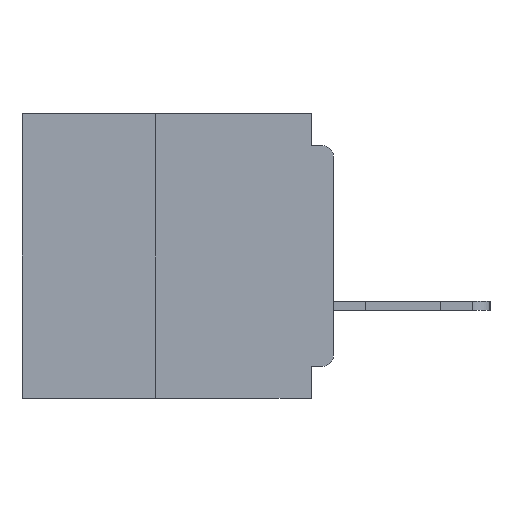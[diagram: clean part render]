
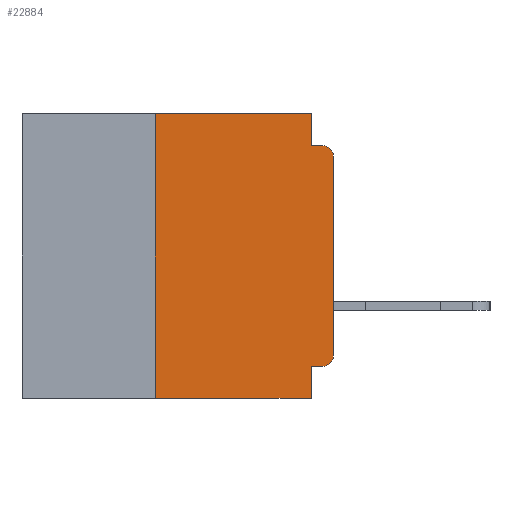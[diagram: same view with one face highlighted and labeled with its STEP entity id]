
A CAD part, left-side view. The second image highlights one B-rep face of the part: STEP entity #22884.
In plain terms, the highlighted planar face has unit normal (-1, 0, 0).
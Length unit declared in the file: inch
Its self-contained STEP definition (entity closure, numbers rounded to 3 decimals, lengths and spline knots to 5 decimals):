
#156 = VECTOR ( 'NONE', #20571, 39.37008 ) ;
#613 = CARTESIAN_POINT ( 'NONE',  ( 0., 0.031, 0. ) ) ;
#863 = ORIENTED_EDGE ( 'NONE', *, *, #7558, .F. ) ;
#2432 = DIRECTION ( 'NONE',  ( 0., -1., 0. ) ) ;
#2804 = LINE ( 'NONE', #26421, #23518 ) ;
#2999 = AXIS2_PLACEMENT_3D ( 'NONE', #21089, #50036, #25255 ) ;
#4055 = CARTESIAN_POINT ( 'NONE',  ( 0., 0., -0.045 ) ) ;
#5027 = PLANE ( 'NONE',  #18846 ) ;
#5218 = DIRECTION ( 'NONE',  ( 1., 0., 0. ) ) ;
#6605 = DIRECTION ( 'NONE',  ( 0., 0., -1. ) ) ;
#7536 = LINE ( 'NONE', #10752, #28291 ) ;
#7558 = EDGE_CURVE ( 'NONE', #16709, #9457, #7536, .T. ) ;
#7922 = VECTOR ( 'NONE', #2432, 39.37008 ) ;
#8011 = DIRECTION ( 'NONE',  ( 0., -1., 0. ) ) ;
#8352 = LINE ( 'NONE', #15480, #40159 ) ;
#8773 = VERTEX_POINT ( 'NONE', #31298 ) ;
#9457 = VERTEX_POINT ( 'NONE', #48027 ) ;
#10752 = CARTESIAN_POINT ( 'NONE',  ( 0., 0.031, 0. ) ) ;
#10824 = VECTOR ( 'NONE', #41363, 39.37008 ) ;
#13518 = EDGE_CURVE ( 'NONE', #9457, #46432, #51888, .T. ) ;
#14701 = VERTEX_POINT ( 'NONE', #28368 ) ;
#15480 = CARTESIAN_POINT ( 'NONE',  ( 0., 0.25, -0.4 ) ) ;
#16709 = VERTEX_POINT ( 'NONE', #613 ) ;
#17668 = LINE ( 'NONE', #27251, #7922 ) ;
#18846 = AXIS2_PLACEMENT_3D ( 'NONE', #30014, #5218, #34219 ) ;
#18885 = VECTOR ( 'NONE', #8011, 39.37008 ) ;
#19050 = CIRCLE ( 'NONE', #39985, 0.015 ) ;
#20107 = VERTEX_POINT ( 'NONE', #28566 ) ;
#20383 = DIRECTION ( 'NONE',  ( 0., 1., 0. ) ) ;
#20571 = DIRECTION ( 'NONE',  ( 0., 0., 1. ) ) ;
#20787 = DIRECTION ( 'NONE',  ( -1., 0., 0. ) ) ;
#21089 = CARTESIAN_POINT ( 'NONE',  ( 0., 0.015, -0.34 ) ) ;
#21862 = LINE ( 'NONE', #53591, #10824 ) ;
#22233 = CARTESIAN_POINT ( 'NONE',  ( 0., 0.031, -0.355 ) ) ;
#22884 = ADVANCED_FACE ( 'NONE', ( #32968 ), #5027, .F. ) ;
#23518 = VECTOR ( 'NONE', #30559, 39.37008 ) ;
#24378 = ORIENTED_EDGE ( 'NONE', *, *, #25657, .T. ) ;
#24441 = ORIENTED_EDGE ( 'NONE', *, *, #44058, .T. ) ;
#25255 = DIRECTION ( 'NONE',  ( 0., 0., -1. ) ) ;
#25657 = EDGE_CURVE ( 'NONE', #14701, #8773, #30044, .T. ) ;
#26421 = CARTESIAN_POINT ( 'NONE',  ( 0., 0.437, -0.4 ) ) ;
#27190 = CARTESIAN_POINT ( 'NONE',  ( 0., 0.031, -0.4 ) ) ;
#27251 = CARTESIAN_POINT ( 'NONE',  ( 0., 0.437, 0. ) ) ;
#28291 = VECTOR ( 'NONE', #6605, 39.37008 ) ;
#28368 = CARTESIAN_POINT ( 'NONE',  ( 0., 0.015, -0.355 ) ) ;
#28566 = CARTESIAN_POINT ( 'NONE',  ( 0., 0.25, -0.4 ) ) ;
#30014 = CARTESIAN_POINT ( 'NONE',  ( 0., 0.437, 0. ) ) ;
#30044 = CIRCLE ( 'NONE', #2999, 0.015 ) ;
#30559 = DIRECTION ( 'NONE',  ( 0., -1., 0. ) ) ;
#31222 = EDGE_CURVE ( 'NONE', #33721, #46432, #19050, .T. ) ;
#31298 = CARTESIAN_POINT ( 'NONE',  ( 0., 0., -0.34 ) ) ;
#32103 = EDGE_CURVE ( 'NONE', #39779, #16709, #17668, .T. ) ;
#32968 = FACE_OUTER_BOUND ( 'NONE', #49665, .T. ) ;
#33270 = LINE ( 'NONE', #49501, #156 ) ;
#33574 = ORIENTED_EDGE ( 'NONE', *, *, #33623, .F. ) ;
#33623 = EDGE_CURVE ( 'NONE', #49928, #47653, #21862, .T. ) ;
#33721 = VERTEX_POINT ( 'NONE', #42089 ) ;
#34219 = DIRECTION ( 'NONE',  ( 0., 0., -1. ) ) ;
#37484 = CARTESIAN_POINT ( 'NONE',  ( 0., 0.015, -0.045 ) ) ;
#39779 = VERTEX_POINT ( 'NONE', #46089 ) ;
#39985 = AXIS2_PLACEMENT_3D ( 'NONE', #45619, #20787, #49726 ) ;
#40159 = VECTOR ( 'NONE', #41024, 39.37008 ) ;
#41024 = DIRECTION ( 'NONE',  ( 0., 0., 1. ) ) ;
#41363 = DIRECTION ( 'NONE',  ( 0., 0., -1. ) ) ;
#42089 = CARTESIAN_POINT ( 'NONE',  ( 0., 0., -0.06 ) ) ;
#42483 = ORIENTED_EDGE ( 'NONE', *, *, #50218, .F. ) ;
#43562 = ORIENTED_EDGE ( 'NONE', *, *, #31222, .T. ) ;
#44050 = ORIENTED_EDGE ( 'NONE', *, *, #32103, .F. ) ;
#44058 = EDGE_CURVE ( 'NONE', #8773, #33721, #33270, .T. ) ;
#44704 = EDGE_CURVE ( 'NONE', #20107, #47653, #2804, .T. ) ;
#45106 = EDGE_CURVE ( 'NONE', #14701, #49928, #48061, .T. ) ;
#45619 = CARTESIAN_POINT ( 'NONE',  ( 0., 0.015, -0.06 ) ) ;
#46089 = CARTESIAN_POINT ( 'NONE',  ( 0., 0.25, 0. ) ) ;
#46432 = VERTEX_POINT ( 'NONE', #37484 ) ;
#46786 = VECTOR ( 'NONE', #20383, 39.37008 ) ;
#47491 = ORIENTED_EDGE ( 'NONE', *, *, #13518, .F. ) ;
#47653 = VERTEX_POINT ( 'NONE', #27190 ) ;
#47728 = ORIENTED_EDGE ( 'NONE', *, *, #45106, .F. ) ;
#48027 = CARTESIAN_POINT ( 'NONE',  ( 0., 0.031, -0.045 ) ) ;
#48061 = LINE ( 'NONE', #53446, #46786 ) ;
#48475 = ORIENTED_EDGE ( 'NONE', *, *, #44704, .T. ) ;
#49501 = CARTESIAN_POINT ( 'NONE',  ( 0., 0., 0. ) ) ;
#49665 = EDGE_LOOP ( 'NONE', ( #24441, #43562, #47491, #863, #44050, #42483, #48475, #33574, #47728, #24378 ) ) ;
#49726 = DIRECTION ( 'NONE',  ( 0., 0., -1. ) ) ;
#49928 = VERTEX_POINT ( 'NONE', #22233 ) ;
#50036 = DIRECTION ( 'NONE',  ( -1., 0., 0. ) ) ;
#50218 = EDGE_CURVE ( 'NONE', #20107, #39779, #8352, .T. ) ;
#51888 = LINE ( 'NONE', #4055, #18885 ) ;
#53446 = CARTESIAN_POINT ( 'NONE',  ( 0., 0., -0.355 ) ) ;
#53591 = CARTESIAN_POINT ( 'NONE',  ( 0., 0.031, -0.4 ) ) ;
